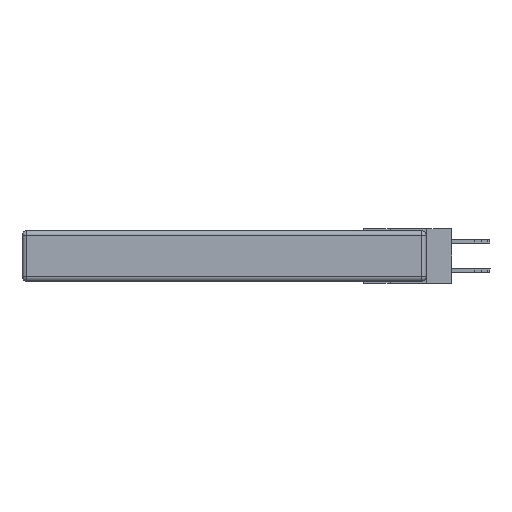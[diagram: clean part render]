
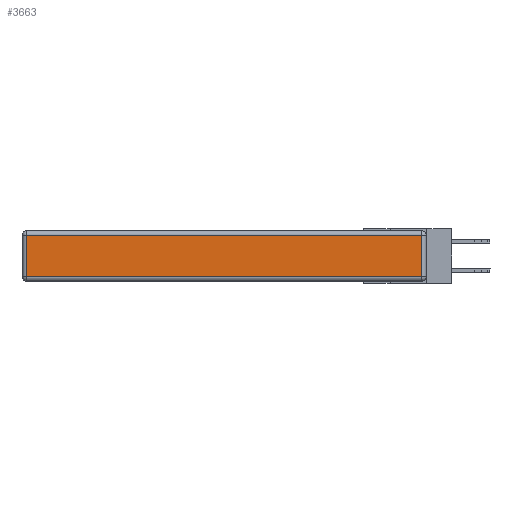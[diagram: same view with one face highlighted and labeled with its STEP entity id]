
A CAD part, left-side view. The second image highlights one B-rep face of the part: STEP entity #3663.
In plain terms, the highlighted planar face has unit normal (-1, 0, 0).
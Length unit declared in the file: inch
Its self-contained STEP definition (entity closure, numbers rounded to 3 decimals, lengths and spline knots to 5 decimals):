
#424 = DIRECTION ( 'NONE',  ( -1., 0., 0. ) ) ;
#752 = CARTESIAN_POINT ( 'NONE',  ( 0., 0.03, -0.03 ) ) ;
#1215 = LINE ( 'NONE', #3668, #7385 ) ;
#2758 = EDGE_CURVE ( 'NONE', #15455, #9835, #8858, .T. ) ;
#2896 = CARTESIAN_POINT ( 'NONE',  ( 0., 0., -0.343 ) ) ;
#3010 = CARTESIAN_POINT ( 'NONE',  ( 0., 0., -0.313 ) ) ;
#3314 = CARTESIAN_POINT ( 'NONE',  ( 0., 0.03, -0.343 ) ) ;
#3508 = EDGE_LOOP ( 'NONE', ( #6333, #15610, #14953, #3732 ) ) ;
#3663 = ADVANCED_FACE ( 'NONE', ( #15627 ), #5356, .T. ) ;
#3668 = CARTESIAN_POINT ( 'NONE',  ( 0., 2.72, -0.343 ) ) ;
#3732 = ORIENTED_EDGE ( 'NONE', *, *, #9522, .T. ) ;
#3948 = LINE ( 'NONE', #3010, #14629 ) ;
#4069 = DIRECTION ( 'NONE',  ( 0., -1., 0. ) ) ;
#4777 = VECTOR ( 'NONE', #14244, 39.37008 ) ;
#5356 = PLANE ( 'NONE',  #11144 ) ;
#5564 = EDGE_CURVE ( 'NONE', #9835, #14587, #13313, .T. ) ;
#6193 = CARTESIAN_POINT ( 'NONE',  ( 0., 2.72, -0.03 ) ) ;
#6333 = ORIENTED_EDGE ( 'NONE', *, *, #11977, .T. ) ;
#7095 = VECTOR ( 'NONE', #12493, 39.37008 ) ;
#7385 = VECTOR ( 'NONE', #12334, 39.37008 ) ;
#7434 = CARTESIAN_POINT ( 'NONE',  ( 0., 2.72, -0.313 ) ) ;
#8858 = LINE ( 'NONE', #3314, #4777 ) ;
#9522 = EDGE_CURVE ( 'NONE', #14587, #15057, #1215, .T. ) ;
#9835 = VERTEX_POINT ( 'NONE', #752 ) ;
#11144 = AXIS2_PLACEMENT_3D ( 'NONE', #2896, #424, #11407 ) ;
#11407 = DIRECTION ( 'NONE',  ( 0., 0., 1. ) ) ;
#11977 = EDGE_CURVE ( 'NONE', #15057, #15455, #3948, .T. ) ;
#12334 = DIRECTION ( 'NONE',  ( 0., 0., -1. ) ) ;
#12493 = DIRECTION ( 'NONE',  ( 0., 1., 0. ) ) ;
#13313 = LINE ( 'NONE', #14619, #7095 ) ;
#13762 = CARTESIAN_POINT ( 'NONE',  ( 0., 0.03, -0.313 ) ) ;
#14244 = DIRECTION ( 'NONE',  ( 0., 0., 1. ) ) ;
#14587 = VERTEX_POINT ( 'NONE', #6193 ) ;
#14619 = CARTESIAN_POINT ( 'NONE',  ( 0., 2.75, -0.03 ) ) ;
#14629 = VECTOR ( 'NONE', #4069, 39.37008 ) ;
#14953 = ORIENTED_EDGE ( 'NONE', *, *, #5564, .T. ) ;
#15057 = VERTEX_POINT ( 'NONE', #7434 ) ;
#15455 = VERTEX_POINT ( 'NONE', #13762 ) ;
#15610 = ORIENTED_EDGE ( 'NONE', *, *, #2758, .T. ) ;
#15627 = FACE_OUTER_BOUND ( 'NONE', #3508, .T. ) ;
